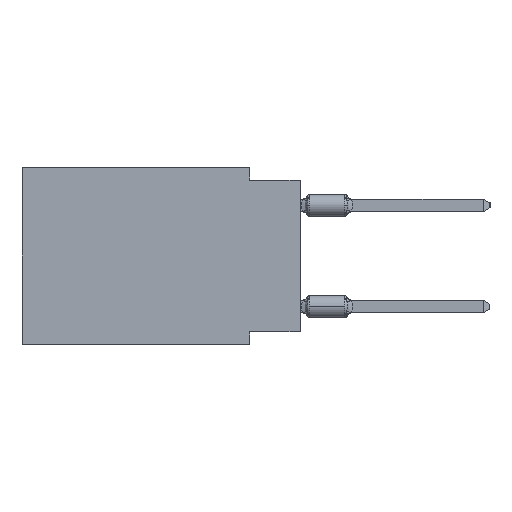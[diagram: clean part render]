
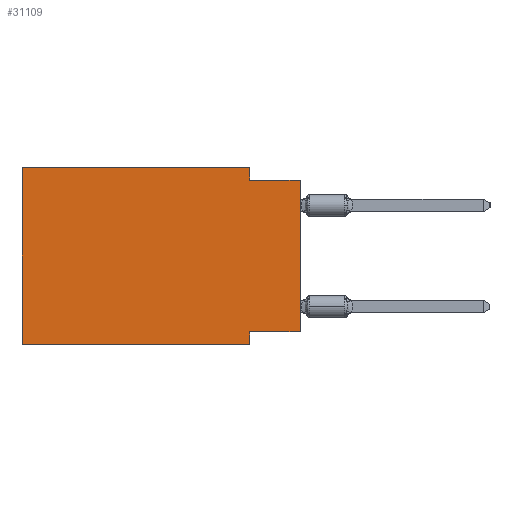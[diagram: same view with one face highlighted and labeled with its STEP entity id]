
A CAD part, left-side view. The second image highlights one B-rep face of the part: STEP entity #31109.
In plain terms, the highlighted planar face has unit normal (-1, 0, 0).
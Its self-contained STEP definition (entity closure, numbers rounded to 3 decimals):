
#752 = LINE ( 'NONE', #3235, #26067 ) ;
#1230 = LINE ( 'NONE', #33565, #26994 ) ;
#2458 = PLANE ( 'NONE',  #15079 ) ;
#2743 = LINE ( 'NONE', #10820, #30481 ) ;
#3235 = CARTESIAN_POINT ( 'NONE',  ( 0., 13.97, 0. ) ) ;
#3356 = DIRECTION ( 'NONE',  ( 0., -1., 0. ) ) ;
#3609 = ORIENTED_EDGE ( 'NONE', *, *, #4471, .F. ) ;
#3881 = ORIENTED_EDGE ( 'NONE', *, *, #22676, .F. ) ;
#4471 = EDGE_CURVE ( 'NONE', #27130, #16990, #6762, .T. ) ;
#4557 = CARTESIAN_POINT ( 'NONE',  ( 0., 0., 0. ) ) ;
#5130 = FACE_OUTER_BOUND ( 'NONE', #7804, .T. ) ;
#5836 = LINE ( 'NONE', #25033, #32871 ) ;
#6133 = VECTOR ( 'NONE', #26239, 1000. ) ;
#6446 = EDGE_CURVE ( 'NONE', #22340, #12575, #2743, .T. ) ;
#6762 = LINE ( 'NONE', #33594, #12300 ) ;
#6877 = LINE ( 'NONE', #4557, #6133 ) ;
#7804 = EDGE_LOOP ( 'NONE', ( #18273, #8013, #18333, #10966, #12057, #18705, #3609, #3881 ) ) ;
#8013 = ORIENTED_EDGE ( 'NONE', *, *, #6446, .F. ) ;
#9012 = EDGE_CURVE ( 'NONE', #23660, #10595, #752, .T. ) ;
#9642 = LINE ( 'NONE', #14636, #14703 ) ;
#9734 = VECTOR ( 'NONE', #20260, 1000. ) ;
#10595 = VERTEX_POINT ( 'NONE', #28443 ) ;
#10820 = CARTESIAN_POINT ( 'NONE',  ( 0., 0., -0.635 ) ) ;
#10966 = ORIENTED_EDGE ( 'NONE', *, *, #9012, .F. ) ;
#11531 = CARTESIAN_POINT ( 'NONE',  ( 0., 2.54, -8.255 ) ) ;
#12057 = ORIENTED_EDGE ( 'NONE', *, *, #21532, .F. ) ;
#12147 = CARTESIAN_POINT ( 'NONE',  ( 0., 2.54, -8.89 ) ) ;
#12270 = DIRECTION ( 'NONE',  ( 0., 0., -1. ) ) ;
#12300 = VECTOR ( 'NONE', #12270, 1000. ) ;
#12417 = LINE ( 'NONE', #14571, #9734 ) ;
#12575 = VERTEX_POINT ( 'NONE', #22184 ) ;
#13465 = EDGE_CURVE ( 'NONE', #19946, #16990, #12417, .T. ) ;
#14571 = CARTESIAN_POINT ( 'NONE',  ( 0., 13.97, -8.89 ) ) ;
#14636 = CARTESIAN_POINT ( 'NONE',  ( 0., 0., -8.255 ) ) ;
#14703 = VECTOR ( 'NONE', #28306, 1000. ) ;
#15079 = AXIS2_PLACEMENT_3D ( 'NONE', #34962, #21493, #22190 ) ;
#16990 = VERTEX_POINT ( 'NONE', #12147 ) ;
#17848 = EDGE_CURVE ( 'NONE', #10595, #22340, #1230, .T. ) ;
#18273 = ORIENTED_EDGE ( 'NONE', *, *, #22438, .T. ) ;
#18333 = ORIENTED_EDGE ( 'NONE', *, *, #17848, .F. ) ;
#18705 = ORIENTED_EDGE ( 'NONE', *, *, #13465, .T. ) ;
#19946 = VERTEX_POINT ( 'NONE', #22066 ) ;
#20055 = CARTESIAN_POINT ( 'NONE',  ( 0., 2.54, -0.635 ) ) ;
#20260 = DIRECTION ( 'NONE',  ( 0., -1., 0. ) ) ;
#21493 = DIRECTION ( 'NONE',  ( 1., 0., 0. ) ) ;
#21532 = EDGE_CURVE ( 'NONE', #19946, #23660, #5836, .T. ) ;
#22066 = CARTESIAN_POINT ( 'NONE',  ( 0., 13.97, -8.89 ) ) ;
#22184 = CARTESIAN_POINT ( 'NONE',  ( 0., 0., -0.635 ) ) ;
#22190 = DIRECTION ( 'NONE',  ( 0., 0., -1. ) ) ;
#22340 = VERTEX_POINT ( 'NONE', #20055 ) ;
#22396 = DIRECTION ( 'NONE',  ( 0., 0., -1. ) ) ;
#22438 = EDGE_CURVE ( 'NONE', #27666, #12575, #6877, .T. ) ;
#22676 = EDGE_CURVE ( 'NONE', #27666, #27130, #9642, .T. ) ;
#23660 = VERTEX_POINT ( 'NONE', #28729 ) ;
#25033 = CARTESIAN_POINT ( 'NONE',  ( 0., 13.97, 0. ) ) ;
#26067 = VECTOR ( 'NONE', #27395, 1000. ) ;
#26239 = DIRECTION ( 'NONE',  ( 0., 0., 1. ) ) ;
#26994 = VECTOR ( 'NONE', #22396, 1000. ) ;
#27130 = VERTEX_POINT ( 'NONE', #11531 ) ;
#27395 = DIRECTION ( 'NONE',  ( 0., -1., 0. ) ) ;
#27666 = VERTEX_POINT ( 'NONE', #28150 ) ;
#28150 = CARTESIAN_POINT ( 'NONE',  ( 0., 0., -8.255 ) ) ;
#28306 = DIRECTION ( 'NONE',  ( 0., 1., 0. ) ) ;
#28443 = CARTESIAN_POINT ( 'NONE',  ( 0., 2.54, 0. ) ) ;
#28729 = CARTESIAN_POINT ( 'NONE',  ( 0., 13.97, 0. ) ) ;
#30481 = VECTOR ( 'NONE', #3356, 1000. ) ;
#30873 = DIRECTION ( 'NONE',  ( 0., 0., 1. ) ) ;
#31109 = ADVANCED_FACE ( 'NONE', ( #5130 ), #2458, .F. ) ;
#32871 = VECTOR ( 'NONE', #30873, 1000. ) ;
#33565 = CARTESIAN_POINT ( 'NONE',  ( 0., 2.54, 0. ) ) ;
#33594 = CARTESIAN_POINT ( 'NONE',  ( 0., 2.54, -8.89 ) ) ;
#34962 = CARTESIAN_POINT ( 'NONE',  ( 0., 13.97, 0. ) ) ;
